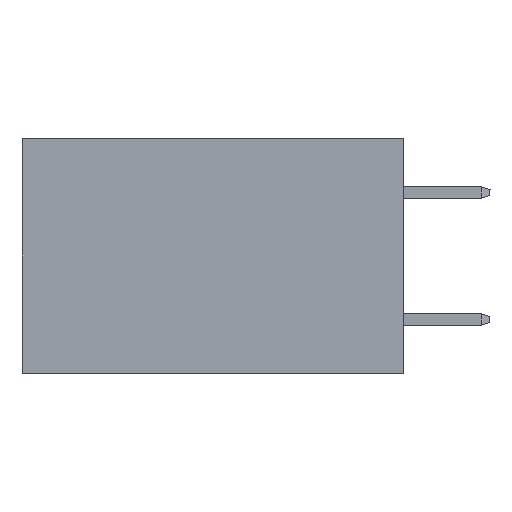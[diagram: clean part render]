
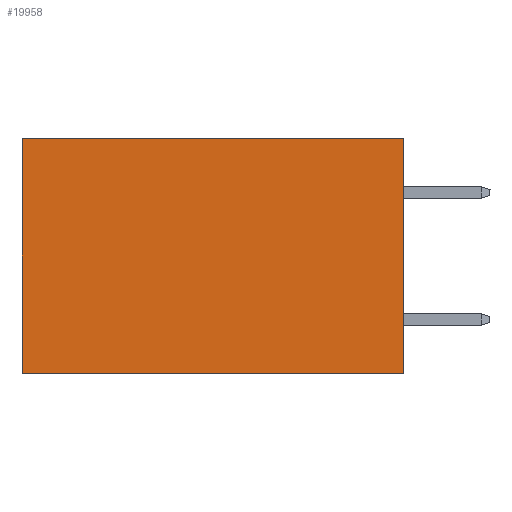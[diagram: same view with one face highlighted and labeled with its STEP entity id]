
A CAD part, left-side view. The second image highlights one B-rep face of the part: STEP entity #19958.
In plain terms, the highlighted planar face has unit normal (-1, 0, 0).
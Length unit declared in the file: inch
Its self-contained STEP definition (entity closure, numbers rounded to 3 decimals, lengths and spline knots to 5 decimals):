
#2201 = EDGE_CURVE ( 'NONE', #25252, #27754, #23564, .T. ) ;
#2446 = VECTOR ( 'NONE', #13729, 39.37008 ) ;
#2889 = CARTESIAN_POINT ( 'NONE',  ( 0.2875, 0.6, 0. ) ) ;
#3346 = AXIS2_PLACEMENT_3D ( 'NONE', #33770, #10610, #23935 ) ;
#3739 = ORIENTED_EDGE ( 'NONE', *, *, #21481, .F. ) ;
#4064 = VECTOR ( 'NONE', #11605, 39.37008 ) ;
#5756 = DIRECTION ( 'NONE',  ( 0., 1., 0. ) ) ;
#8912 = VERTEX_POINT ( 'NONE', #11893 ) ;
#10386 = PLANE ( 'NONE',  #3346 ) ;
#10610 = DIRECTION ( 'NONE',  ( 1., 0., 0. ) ) ;
#11605 = DIRECTION ( 'NONE',  ( 0., 1., 0. ) ) ;
#11893 = CARTESIAN_POINT ( 'NONE',  ( 0.2875, 0.6, 0. ) ) ;
#13671 = FACE_OUTER_BOUND ( 'NONE', #40624, .T. ) ;
#13729 = DIRECTION ( 'NONE',  ( 0., 0., -1. ) ) ;
#14072 = EDGE_CURVE ( 'NONE', #25252, #8912, #15821, .T. ) ;
#15821 = LINE ( 'NONE', #22367, #29572 ) ;
#16646 = LINE ( 'NONE', #2889, #22766 ) ;
#19958 = ADVANCED_FACE ( 'NONE', ( #13671 ), #10386, .F. ) ;
#21216 = CARTESIAN_POINT ( 'NONE',  ( 0.2875, 0., -0.37 ) ) ;
#21481 = EDGE_CURVE ( 'NONE', #27754, #25559, #21854, .T. ) ;
#21854 = LINE ( 'NONE', #21216, #4064 ) ;
#22367 = CARTESIAN_POINT ( 'NONE',  ( 0.2875, 0., 0. ) ) ;
#22766 = VECTOR ( 'NONE', #33262, 39.37008 ) ;
#23564 = LINE ( 'NONE', #36902, #2446 ) ;
#23935 = DIRECTION ( 'NONE',  ( 0., 0., -1. ) ) ;
#24936 = ORIENTED_EDGE ( 'NONE', *, *, #41489, .T. ) ;
#25252 = VERTEX_POINT ( 'NONE', #30670 ) ;
#25559 = VERTEX_POINT ( 'NONE', #33777 ) ;
#27754 = VERTEX_POINT ( 'NONE', #41121 ) ;
#29572 = VECTOR ( 'NONE', #5756, 39.37008 ) ;
#30670 = CARTESIAN_POINT ( 'NONE',  ( 0.2875, 0., 0. ) ) ;
#30947 = ORIENTED_EDGE ( 'NONE', *, *, #14072, .T. ) ;
#33262 = DIRECTION ( 'NONE',  ( 0., 0., -1. ) ) ;
#33770 = CARTESIAN_POINT ( 'NONE',  ( 0.2875, 0., 0. ) ) ;
#33777 = CARTESIAN_POINT ( 'NONE',  ( 0.2875, 0.6, -0.37 ) ) ;
#36902 = CARTESIAN_POINT ( 'NONE',  ( 0.2875, 0., 0. ) ) ;
#40624 = EDGE_LOOP ( 'NONE', ( #24936, #3739, #42551, #30947 ) ) ;
#41121 = CARTESIAN_POINT ( 'NONE',  ( 0.2875, 0., -0.37 ) ) ;
#41489 = EDGE_CURVE ( 'NONE', #8912, #25559, #16646, .T. ) ;
#42551 = ORIENTED_EDGE ( 'NONE', *, *, #2201, .F. ) ;
